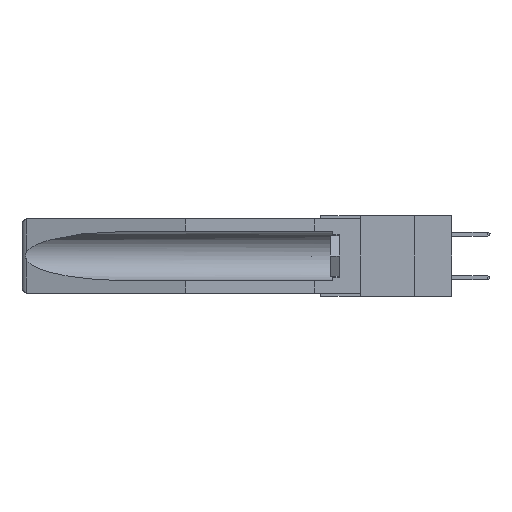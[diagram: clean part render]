
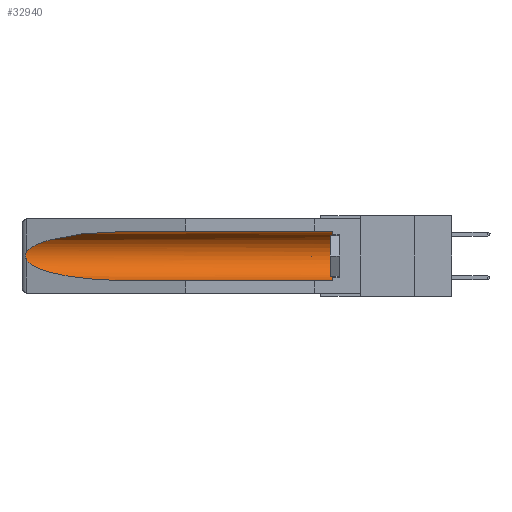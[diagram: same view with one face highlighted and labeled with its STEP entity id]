
A CAD part, left-side view. The second image highlights one B-rep face of the part: STEP entity #32940.
In plain terms, the highlighted cylindrical face has radius 2.857 mm (diameter 5.715 mm), a partial arc.
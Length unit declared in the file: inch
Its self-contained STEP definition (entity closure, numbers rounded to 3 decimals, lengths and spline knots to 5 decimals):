
#510 = VERTEX_POINT ( 'NONE', #23051 ) ;
#717 = DIRECTION ( 'NONE',  ( 0., 0., 1. ) ) ;
#814 = EDGE_CURVE ( 'NONE', #14985, #34826, #12531, .T. ) ;
#2416 = ORIENTED_EDGE ( 'NONE', *, *, #814, .F. ) ;
#2675 = CARTESIAN_POINT ( 'NONE',  ( 0.155, -0.30754, -0.1715 ) ) ;
#2972 = LINE ( 'NONE', #16017, #22536 ) ;
#3406 = CARTESIAN_POINT ( 'NONE',  ( 0.155, 0.126, -0.284 ) ) ;
#3623 = EDGE_CURVE ( 'NONE', #23266, #34826, #16364, .T. ) ;
#4695 = CYLINDRICAL_SURFACE ( 'NONE', #20255, 0.1125 ) ;
#5491 = ORIENTED_EDGE ( 'NONE', *, *, #26882, .T. ) ;
#5673 = EDGE_LOOP ( 'NONE', ( #23627, #17606, #8620, #2416, #5491, #10683 ) ) ;
#7045 = CARTESIAN_POINT ( 'NONE',  ( 0.155, 1.07973, -0.284 ) ) ;
#7643 = CARTESIAN_POINT ( 'NONE',  ( 0.155, 1.07973, -0.059 ) ) ;
#7943 = CARTESIAN_POINT ( 'NONE',  ( 0.155, 0.126, -0.1715 ) ) ;
#8585 = EDGE_CURVE ( 'NONE', #510, #13913, #25212, .T. ) ;
#8620 = ORIENTED_EDGE ( 'NONE', *, *, #3623, .T. ) ;
#10568 = DIRECTION ( 'NONE',  ( 0., 0., 1. ) ) ;
#10683 = ORIENTED_EDGE ( 'NONE', *, *, #23930, .T. ) ;
#12217 = CARTESIAN_POINT ( 'NONE',  ( 0.155, 1.07973, -0.284 ) ) ;
#12428 = DIRECTION ( 'NONE',  ( 0., 1., 0. ) ) ;
#12531 = LINE ( 'NONE', #26245, #18520 ) ;
#12721 = FACE_OUTER_BOUND ( 'NONE', #5673, .T. ) ;
#13215 = CARTESIAN_POINT ( 'NONE',  ( 0.26537, 1.52718, -0.19328 ) ) ;
#13392 = CIRCLE ( 'NONE', #24687, 0.1125 ) ;
#13714 = DIRECTION ( 'NONE',  ( 0., 1., 0. ) ) ;
#13913 = VERTEX_POINT ( 'NONE', #31372 ) ;
#14985 = VERTEX_POINT ( 'NONE', #3406 ) ;
#15334 = CARTESIAN_POINT ( 'NONE',  ( 0.2673, 1.53269, -0.17917 ) ) ;
#15564 = CARTESIAN_POINT ( 'NONE',  ( 0.26597, 1.5296, -0.19026 ) ) ;
#16017 = CARTESIAN_POINT ( 'NONE',  ( 0.155, -0.30754, -0.059 ) ) ;
#16364 =( BOUNDED_CURVE ( )  B_SPLINE_CURVE ( 3, ( #34182, #23315, #26435, #7045 ),
 .UNSPECIFIED., .F., .T. ) 
 B_SPLINE_CURVE_WITH_KNOTS ( ( 4, 4 ),
 ( 0.1948, 1.5708 ),
 .UNSPECIFIED. ) 
 CURVE ( )  GEOMETRIC_REPRESENTATION_ITEM ( )  RATIONAL_B_SPLINE_CURVE ( ( 1., 0.848, 0.848, 1. ) ) 
 REPRESENTATION_ITEM ( '' )  );
#17606 = ORIENTED_EDGE ( 'NONE', *, *, #24495, .T. ) ;
#18261 = DIRECTION ( 'NONE',  ( 0., 1., 0. ) ) ;
#18520 = VECTOR ( 'NONE', #18261, 39.37008 ) ;
#18531 = DIRECTION ( 'NONE',  ( 0., -1., 0. ) ) ;
#19827 = CARTESIAN_POINT ( 'NONE',  ( 0.26537, 1.52718, -0.14972 ) ) ;
#20255 = AXIS2_PLACEMENT_3D ( 'NONE', #2675, #13714, #717 ) ;
#20916 = CARTESIAN_POINT ( 'NONE',  ( 0.2673, 1.5327, -0.16383 ) ) ;
#21036 = CARTESIAN_POINT ( 'NONE',  ( 0.26537, 1.52718, -0.19328 ) ) ;
#22536 = VECTOR ( 'NONE', #12428, 39.37008 ) ;
#23051 = CARTESIAN_POINT ( 'NONE',  ( 0.155, 1.07973, -0.059 ) ) ;
#23266 = VERTEX_POINT ( 'NONE', #13215 ) ;
#23315 = CARTESIAN_POINT ( 'NONE',  ( 0.25451, 1.48313, -0.24835 ) ) ;
#23627 = ORIENTED_EDGE ( 'NONE', *, *, #8585, .T. ) ;
#23930 = EDGE_CURVE ( 'NONE', #29310, #510, #2972, .T. ) ;
#24495 = EDGE_CURVE ( 'NONE', #13913, #23266, #34396, .T. ) ;
#24687 = AXIS2_PLACEMENT_3D ( 'NONE', #7943, #18531, #10568 ) ;
#25212 =( BOUNDED_CURVE ( )  B_SPLINE_CURVE ( 3, ( #7643, #29404, #26780, #26673 ),
 .UNSPECIFIED., .F., .F. ) 
 B_SPLINE_CURVE_WITH_KNOTS ( ( 4, 4 ),
 ( 4.71239, 6.08839 ),
 .UNSPECIFIED. ) 
 CURVE ( )  GEOMETRIC_REPRESENTATION_ITEM ( )  RATIONAL_B_SPLINE_CURVE ( ( 1., 0.848, 0.848, 1. ) ) 
 REPRESENTATION_ITEM ( '' )  );
#26245 = CARTESIAN_POINT ( 'NONE',  ( 0.155, -0.30754, -0.284 ) ) ;
#26398 = CARTESIAN_POINT ( 'NONE',  ( 0.26654, 1.53092, -0.15636 ) ) ;
#26435 = CARTESIAN_POINT ( 'NONE',  ( 0.21114, 1.30732, -0.284 ) ) ;
#26673 = CARTESIAN_POINT ( 'NONE',  ( 0.26537, 1.52718, -0.14972 ) ) ;
#26780 = CARTESIAN_POINT ( 'NONE',  ( 0.25451, 1.48313, -0.09465 ) ) ;
#26882 = EDGE_CURVE ( 'NONE', #14985, #29310, #13392, .T. ) ;
#29126 = CARTESIAN_POINT ( 'NONE',  ( 0.2675, 1.53308, -0.17534 ) ) ;
#29310 = VERTEX_POINT ( 'NONE', #30481 ) ;
#29404 = CARTESIAN_POINT ( 'NONE',  ( 0.21114, 1.30732, -0.059 ) ) ;
#30481 = CARTESIAN_POINT ( 'NONE',  ( 0.155, 0.126, -0.059 ) ) ;
#31024 = CARTESIAN_POINT ( 'NONE',  ( 0.26597, 1.52961, -0.15275 ) ) ;
#31372 = CARTESIAN_POINT ( 'NONE',  ( 0.26537, 1.52718, -0.14972 ) ) ;
#31629 = CARTESIAN_POINT ( 'NONE',  ( 0.2675, 1.53308, -0.16763 ) ) ;
#31868 = CARTESIAN_POINT ( 'NONE',  ( 0.26655, 1.53094, -0.18657 ) ) ;
#32940 = ADVANCED_FACE ( 'NONE', ( #12721 ), #4695, .F. ) ;
#34182 = CARTESIAN_POINT ( 'NONE',  ( 0.26537, 1.52718, -0.19328 ) ) ;
#34396 = B_SPLINE_CURVE_WITH_KNOTS ( 'NONE', 3,
 ( #19827, #31024, #26398, #20916, #31629, #29126, #15334, #31868, #15564, #21036 ),
 .UNSPECIFIED., .F., .F.,
 ( 4, 2, 2, 2, 4 ),
 ( 0., 0.00029, 0.00058, 0.00087, 0.00117 ),
 .UNSPECIFIED. ) ;
#34826 = VERTEX_POINT ( 'NONE', #12217 ) ;
